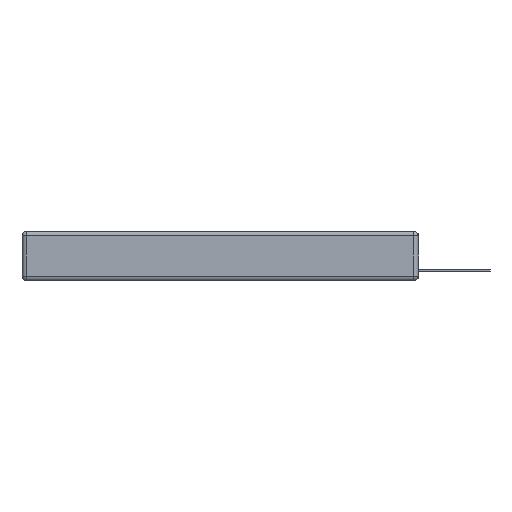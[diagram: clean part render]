
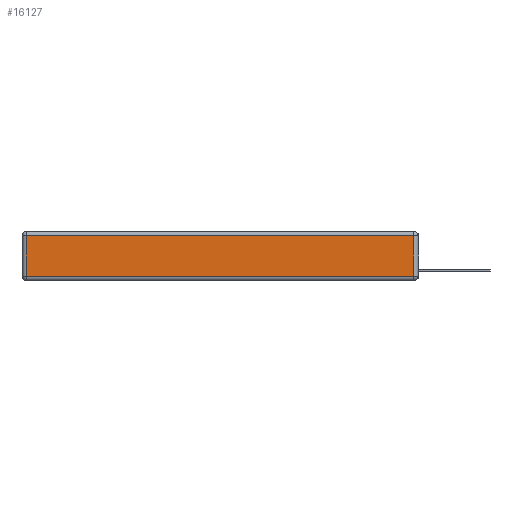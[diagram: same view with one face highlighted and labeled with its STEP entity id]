
A CAD part, left-side view. The second image highlights one B-rep face of the part: STEP entity #16127.
In plain terms, the highlighted planar face has unit normal (-1, 0, 0).
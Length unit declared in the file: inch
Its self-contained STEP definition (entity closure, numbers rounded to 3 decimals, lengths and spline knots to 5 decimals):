
#42 = VERTEX_POINT ( 'NONE', #12894 ) ;
#298 = LINE ( 'NONE', #2681, #3382 ) ;
#1094 = VERTEX_POINT ( 'NONE', #6572 ) ;
#1125 = DIRECTION ( 'NONE',  ( 0., -1., 0. ) ) ;
#1173 = EDGE_CURVE ( 'NONE', #42, #10373, #8342, .T. ) ;
#1751 = DIRECTION ( 'NONE',  ( 0., 0., -1. ) ) ;
#2065 = AXIS2_PLACEMENT_3D ( 'NONE', #9236, #9323, #2896 ) ;
#2524 = CARTESIAN_POINT ( 'NONE',  ( 0., 2.75, -0.03 ) ) ;
#2549 = CARTESIAN_POINT ( 'NONE',  ( 0., 2.72, -0.313 ) ) ;
#2681 = CARTESIAN_POINT ( 'NONE',  ( 0., 2.72, -0.343 ) ) ;
#2755 = CARTESIAN_POINT ( 'NONE',  ( 0., 0.03, -0.03 ) ) ;
#2896 = DIRECTION ( 'NONE',  ( 0., 0., 1. ) ) ;
#3382 = VECTOR ( 'NONE', #1751, 39.37008 ) ;
#6572 = CARTESIAN_POINT ( 'NONE',  ( 0., 2.72, -0.03 ) ) ;
#6797 = EDGE_LOOP ( 'NONE', ( #11558, #14772, #15154, #7158 ) ) ;
#6945 = EDGE_CURVE ( 'NONE', #10373, #1094, #14100, .T. ) ;
#7158 = ORIENTED_EDGE ( 'NONE', *, *, #14823, .T. ) ;
#7673 = DIRECTION ( 'NONE',  ( 0., 1., 0. ) ) ;
#8204 = PLANE ( 'NONE',  #2065 ) ;
#8247 = VERTEX_POINT ( 'NONE', #2549 ) ;
#8342 = LINE ( 'NONE', #16055, #14872 ) ;
#9236 = CARTESIAN_POINT ( 'NONE',  ( 0., 0., -0.343 ) ) ;
#9323 = DIRECTION ( 'NONE',  ( -1., 0., 0. ) ) ;
#9483 = FACE_OUTER_BOUND ( 'NONE', #6797, .T. ) ;
#10373 = VERTEX_POINT ( 'NONE', #2755 ) ;
#10801 = DIRECTION ( 'NONE',  ( 0., 0., 1. ) ) ;
#10825 = EDGE_CURVE ( 'NONE', #8247, #42, #11533, .T. ) ;
#11386 = VECTOR ( 'NONE', #7673, 39.37008 ) ;
#11533 = LINE ( 'NONE', #12724, #16541 ) ;
#11558 = ORIENTED_EDGE ( 'NONE', *, *, #10825, .T. ) ;
#12724 = CARTESIAN_POINT ( 'NONE',  ( 0., 0., -0.313 ) ) ;
#12894 = CARTESIAN_POINT ( 'NONE',  ( 0., 0.03, -0.313 ) ) ;
#14100 = LINE ( 'NONE', #2524, #11386 ) ;
#14772 = ORIENTED_EDGE ( 'NONE', *, *, #1173, .T. ) ;
#14823 = EDGE_CURVE ( 'NONE', #1094, #8247, #298, .T. ) ;
#14872 = VECTOR ( 'NONE', #10801, 39.37008 ) ;
#15154 = ORIENTED_EDGE ( 'NONE', *, *, #6945, .T. ) ;
#16055 = CARTESIAN_POINT ( 'NONE',  ( 0., 0.03, -0.343 ) ) ;
#16127 = ADVANCED_FACE ( 'NONE', ( #9483 ), #8204, .T. ) ;
#16541 = VECTOR ( 'NONE', #1125, 39.37008 ) ;
